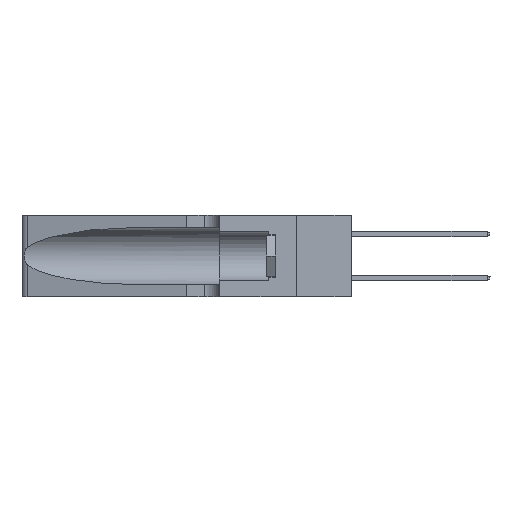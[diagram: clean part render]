
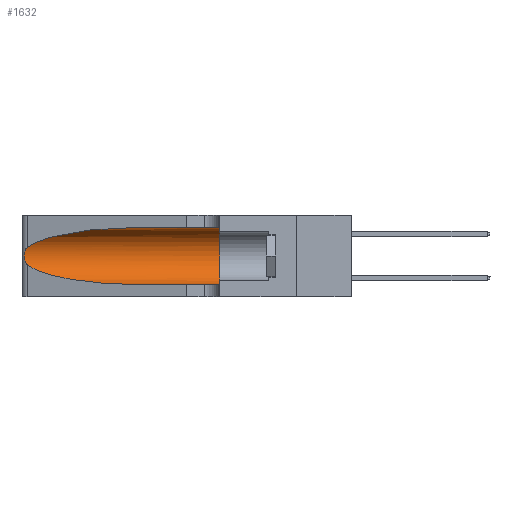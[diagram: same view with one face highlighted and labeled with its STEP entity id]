
A CAD part, left-side view. The second image highlights one B-rep face of the part: STEP entity #1632.
In plain terms, the highlighted cylindrical face has radius 3.308 mm (diameter 6.617 mm), a partial arc.
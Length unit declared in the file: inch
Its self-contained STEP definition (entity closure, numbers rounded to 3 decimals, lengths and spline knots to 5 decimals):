
#84 = CARTESIAN_POINT ( 'NONE',  ( 0.25487, 1.22718, 0.14631 ) ) ;
#366 = EDGE_CURVE ( 'NONE', #18310, #25298, #34889, .T. ) ;
#383 = CARTESIAN_POINT ( 'NONE',  ( 0.25555, 1.22993, 0.14849 ) ) ;
#1096 = DIRECTION ( 'NONE',  ( 0., -1., 0. ) ) ;
#1632 = ADVANCED_FACE ( 'NONE', ( #26397 ), #2227, .F. ) ;
#2227 = CYLINDRICAL_SURFACE ( 'NONE', #19338, 0.13025 ) ;
#2671 = VERTEX_POINT ( 'NONE', #8563 ) ;
#2998 = CARTESIAN_POINT ( 'NONE',  ( 0.26017, 1.23833, 0.17102 ) ) ;
#3419 = CARTESIAN_POINT ( 'NONE',  ( 0.1305, 0.72297, 0.05475 ) ) ;
#3473 = CARTESIAN_POINT ( 'NONE',  ( 0.26075, 1.23896, 0.19203 ) ) ;
#4502 = VERTEX_POINT ( 'NONE', #20288 ) ;
#5267 =( BOUNDED_CURVE ( )  B_SPLINE_CURVE ( 3, ( #84, #23561, #20269, #3419 ),
 .UNSPECIFIED., .F., .T. ) 
 B_SPLINE_CURVE_WITH_KNOTS ( ( 4, 4 ),
 ( 3.44316, 4.71239 ),
 .UNSPECIFIED. ) 
 CURVE ( )  GEOMETRIC_REPRESENTATION_ITEM ( )  RATIONAL_B_SPLINE_CURVE ( ( 1., 0.87, 0.87, 1. ) ) 
 REPRESENTATION_ITEM ( '' )  );
#5809 = CARTESIAN_POINT ( 'NONE',  ( 0.26075, 1.23896, 0.178 ) ) ;
#5929 = CARTESIAN_POINT ( 'NONE',  ( 0.25854, 1.2359, 0.20912 ) ) ;
#6174 = CARTESIAN_POINT ( 'NONE',  ( 0.25789, 1.23486, 0.15765 ) ) ;
#6530 = CARTESIAN_POINT ( 'NONE',  ( 0.1305, 1.61858, 0.31525 ) ) ;
#6885 = CARTESIAN_POINT ( 'NONE',  ( 0.1305, 1.61858, 0.05475 ) ) ;
#6954 = ORIENTED_EDGE ( 'NONE', *, *, #9412, .T. ) ;
#7164 = VECTOR ( 'NONE', #17838, 39.37008 ) ;
#7387 = CARTESIAN_POINT ( 'NONE',  ( 0.1305, 1.61858, 0.185 ) ) ;
#7821 = CARTESIAN_POINT ( 'NONE',  ( 0.1305, 0.72297, 0.31525 ) ) ;
#8030 = CARTESIAN_POINT ( 'NONE',  ( 0.1305, 0.72297, 0.05475 ) ) ;
#8563 = CARTESIAN_POINT ( 'NONE',  ( 0.25487, 1.22718, 0.14631 ) ) ;
#8661 = CARTESIAN_POINT ( 'NONE',  ( 0.2373, 1.15595, 0.28018 ) ) ;
#8685 = ORIENTED_EDGE ( 'NONE', *, *, #15419, .F. ) ;
#9412 = EDGE_CURVE ( 'NONE', #2671, #18310, #5267, .T. ) ;
#12064 = ORIENTED_EDGE ( 'NONE', *, *, #366, .T. ) ;
#12135 = VERTEX_POINT ( 'NONE', #23854 ) ;
#12930 = ORIENTED_EDGE ( 'NONE', *, *, #14815, .T. ) ;
#13406 = CARTESIAN_POINT ( 'NONE',  ( 0.1305, 0.35, 0.185 ) ) ;
#14407 = CARTESIAN_POINT ( 'NONE',  ( 0.25856, 1.23593, 0.16098 ) ) ;
#14751 = CARTESIAN_POINT ( 'NONE',  ( 0.25555, 1.22994, 0.2215 ) ) ;
#14815 = EDGE_CURVE ( 'NONE', #12135, #4502, #16749, .T. ) ;
#15419 = EDGE_CURVE ( 'NONE', #18354, #25298, #31832, .T. ) ;
#15715 = VECTOR ( 'NONE', #1096, 39.37008 ) ;
#16749 =( BOUNDED_CURVE ( )  B_SPLINE_CURVE ( 3, ( #7821, #22302, #8661, #25350 ),
 .UNSPECIFIED., .F., .F. ) 
 B_SPLINE_CURVE_WITH_KNOTS ( ( 4, 4 ),
 ( 1.5708, 2.84003 ),
 .UNSPECIFIED. ) 
 CURVE ( )  GEOMETRIC_REPRESENTATION_ITEM ( )  RATIONAL_B_SPLINE_CURVE ( ( 1., 0.87, 0.87, 1. ) ) 
 REPRESENTATION_ITEM ( '' )  );
#16993 = CARTESIAN_POINT ( 'NONE',  ( 0.25639, 1.23186, 0.15144 ) ) ;
#17110 = CARTESIAN_POINT ( 'NONE',  ( 0.26018, 1.23835, 0.19895 ) ) ;
#17143 = AXIS2_PLACEMENT_3D ( 'NONE', #13406, #33558, #30253 ) ;
#17480 = CARTESIAN_POINT ( 'NONE',  ( 0.25787, 1.23484, 0.2124 ) ) ;
#17838 = DIRECTION ( 'NONE',  ( 0., -1., 0. ) ) ;
#18310 = VERTEX_POINT ( 'NONE', #8030 ) ;
#18354 = VERTEX_POINT ( 'NONE', #33696 ) ;
#19338 = AXIS2_PLACEMENT_3D ( 'NONE', #7387, #29863, #26902 ) ;
#19435 = ORIENTED_EDGE ( 'NONE', *, *, #35105, .T. ) ;
#19827 = CARTESIAN_POINT ( 'NONE',  ( 0.25487, 1.22718, 0.14631 ) ) ;
#20269 = CARTESIAN_POINT ( 'NONE',  ( 0.18966, 0.96281, 0.05475 ) ) ;
#20288 = CARTESIAN_POINT ( 'NONE',  ( 0.25487, 1.22718, 0.22369 ) ) ;
#20384 = B_SPLINE_CURVE_WITH_KNOTS ( 'NONE', 3,
 ( #31621, #14751, #31496, #17480, #5929, #17110, #3473, #5809, #2998, #14407, #6174, #16993, #383, #19827 ),
 .UNSPECIFIED., .F., .F.,
 ( 4, 2, 2, 2, 2, 2, 4 ),
 ( 0., 0.00027, 0.00053, 0.00107, 0.0016, 0.00187, 0.00214 ),
 .UNSPECIFIED. ) ;
#20980 = ORIENTED_EDGE ( 'NONE', *, *, #23039, .F. ) ;
#22302 = CARTESIAN_POINT ( 'NONE',  ( 0.18966, 0.96281, 0.31525 ) ) ;
#22800 = CARTESIAN_POINT ( 'NONE',  ( 0.1305, 0.35, 0.05475 ) ) ;
#23039 = EDGE_CURVE ( 'NONE', #12135, #18354, #23204, .T. ) ;
#23204 = LINE ( 'NONE', #6530, #15715 ) ;
#23561 = CARTESIAN_POINT ( 'NONE',  ( 0.2373, 1.15595, 0.08982 ) ) ;
#23854 = CARTESIAN_POINT ( 'NONE',  ( 0.1305, 0.72297, 0.31525 ) ) ;
#25298 = VERTEX_POINT ( 'NONE', #22800 ) ;
#25350 = CARTESIAN_POINT ( 'NONE',  ( 0.25487, 1.22718, 0.22369 ) ) ;
#26397 = FACE_OUTER_BOUND ( 'NONE', #33636, .T. ) ;
#26902 = DIRECTION ( 'NONE',  ( 0., 0., -1. ) ) ;
#29863 = DIRECTION ( 'NONE',  ( 0., -1., 0. ) ) ;
#30253 = DIRECTION ( 'NONE',  ( 0., 0., 1. ) ) ;
#31496 = CARTESIAN_POINT ( 'NONE',  ( 0.25639, 1.23184, 0.21858 ) ) ;
#31621 = CARTESIAN_POINT ( 'NONE',  ( 0.25487, 1.22718, 0.22369 ) ) ;
#31832 = CIRCLE ( 'NONE', #17143, 0.13025 ) ;
#33558 = DIRECTION ( 'NONE',  ( 0., 1., 0. ) ) ;
#33636 = EDGE_LOOP ( 'NONE', ( #12930, #19435, #6954, #12064, #8685, #20980 ) ) ;
#33696 = CARTESIAN_POINT ( 'NONE',  ( 0.1305, 0.35, 0.31525 ) ) ;
#34889 = LINE ( 'NONE', #6885, #7164 ) ;
#35105 = EDGE_CURVE ( 'NONE', #4502, #2671, #20384, .T. ) ;
